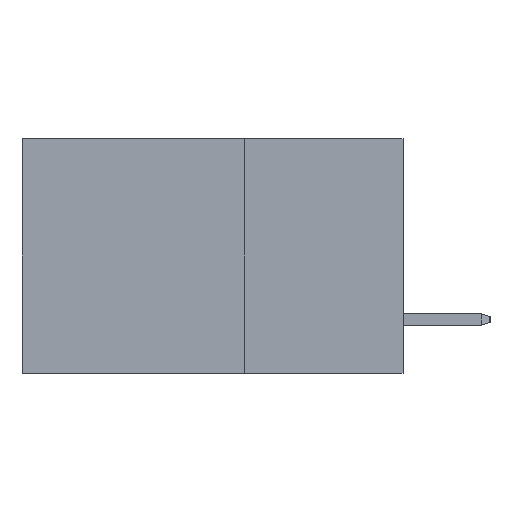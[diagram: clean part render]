
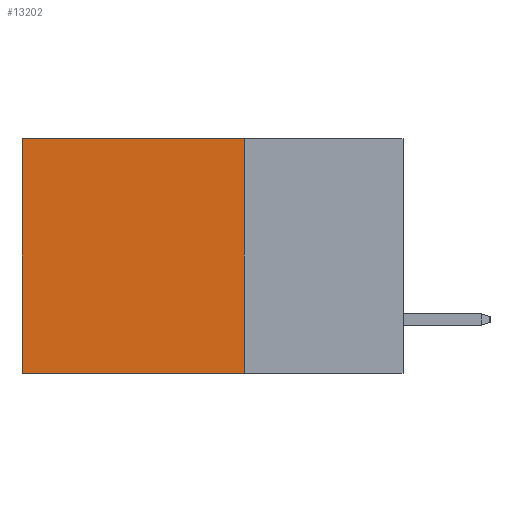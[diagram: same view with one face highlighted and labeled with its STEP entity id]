
A CAD part, left-side view. The second image highlights one B-rep face of the part: STEP entity #13202.
In plain terms, the highlighted planar face has unit normal (-1, 0, 0).
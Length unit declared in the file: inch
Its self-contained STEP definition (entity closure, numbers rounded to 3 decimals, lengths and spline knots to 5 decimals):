
#29 = EDGE_CURVE ( 'NONE', #14675, #396, #11675, .T. ) ;
#58 = CARTESIAN_POINT ( 'NONE',  ( 0.2875, 0.25, -0.37 ) ) ;
#159 = VERTEX_POINT ( 'NONE', #11067 ) ;
#396 = VERTEX_POINT ( 'NONE', #11572 ) ;
#457 = EDGE_CURVE ( 'NONE', #396, #159, #6815, .T. ) ;
#508 = PLANE ( 'NONE',  #15181 ) ;
#1236 = CARTESIAN_POINT ( 'NONE',  ( 0.2875, 0.6, 0. ) ) ;
#1686 = DIRECTION ( 'NONE',  ( 0., 0., -1. ) ) ;
#2929 = LINE ( 'NONE', #15026, #10380 ) ;
#2982 = VECTOR ( 'NONE', #4154, 39.37008 ) ;
#4154 = DIRECTION ( 'NONE',  ( 0., 0., -1. ) ) ;
#5549 = DIRECTION ( 'NONE',  ( 0., 1., 0. ) ) ;
#6815 = LINE ( 'NONE', #1236, #2982 ) ;
#8417 = VECTOR ( 'NONE', #9046, 39.37008 ) ;
#9046 = DIRECTION ( 'NONE',  ( 0., 1., 0. ) ) ;
#9284 = VECTOR ( 'NONE', #5549, 39.37008 ) ;
#9481 = ORIENTED_EDGE ( 'NONE', *, *, #29, .T. ) ;
#9812 = DIRECTION ( 'NONE',  ( 0., 0., -1. ) ) ;
#9981 = ORIENTED_EDGE ( 'NONE', *, *, #13654, .F. ) ;
#10016 = EDGE_LOOP ( 'NONE', ( #10744, #9981, #13042, #9481 ) ) ;
#10380 = VECTOR ( 'NONE', #1686, 39.37008 ) ;
#10744 = ORIENTED_EDGE ( 'NONE', *, *, #457, .T. ) ;
#11067 = CARTESIAN_POINT ( 'NONE',  ( 0.2875, 0.6, -0.37 ) ) ;
#11488 = EDGE_CURVE ( 'NONE', #14675, #15443, #2929, .T. ) ;
#11572 = CARTESIAN_POINT ( 'NONE',  ( 0.2875, 0.6, 0. ) ) ;
#11675 = LINE ( 'NONE', #15752, #8417 ) ;
#11855 = CARTESIAN_POINT ( 'NONE',  ( 0.2875, 0.25, -0.37 ) ) ;
#12168 = LINE ( 'NONE', #58, #9284 ) ;
#13042 = ORIENTED_EDGE ( 'NONE', *, *, #11488, .F. ) ;
#13202 = ADVANCED_FACE ( 'NONE', ( #15100 ), #508, .F. ) ;
#13654 = EDGE_CURVE ( 'NONE', #15443, #159, #12168, .T. ) ;
#13779 = DIRECTION ( 'NONE',  ( 1., 0., 0. ) ) ;
#14675 = VERTEX_POINT ( 'NONE', #15620 ) ;
#15026 = CARTESIAN_POINT ( 'NONE',  ( 0.2875, 0.25, 0. ) ) ;
#15100 = FACE_OUTER_BOUND ( 'NONE', #10016, .T. ) ;
#15181 = AXIS2_PLACEMENT_3D ( 'NONE', #15279, #13779, #9812 ) ;
#15279 = CARTESIAN_POINT ( 'NONE',  ( 0.2875, 0.25, 0. ) ) ;
#15443 = VERTEX_POINT ( 'NONE', #11855 ) ;
#15620 = CARTESIAN_POINT ( 'NONE',  ( 0.2875, 0.25, 0. ) ) ;
#15752 = CARTESIAN_POINT ( 'NONE',  ( 0.2875, 0.25, 0. ) ) ;
